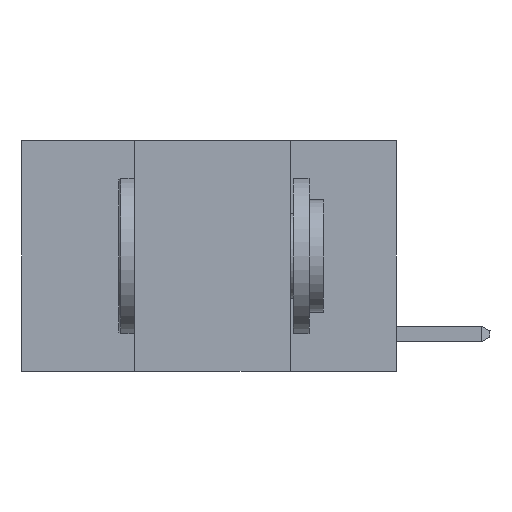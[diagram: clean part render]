
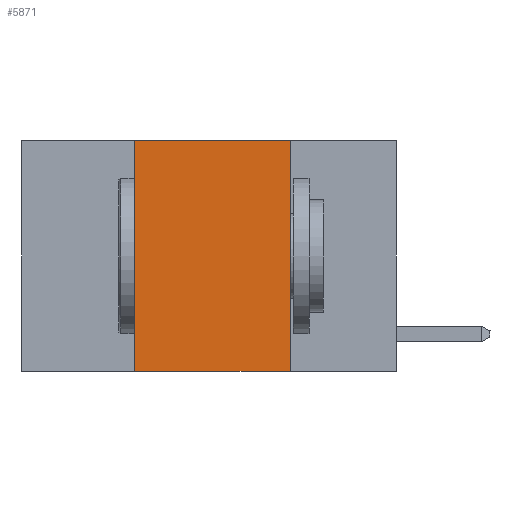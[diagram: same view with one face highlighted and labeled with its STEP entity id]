
A CAD part, left-side view. The second image highlights one B-rep face of the part: STEP entity #5871.
In plain terms, the highlighted planar face has unit normal (-1, 0, 0).
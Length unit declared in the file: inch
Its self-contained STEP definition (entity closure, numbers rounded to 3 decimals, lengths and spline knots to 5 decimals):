
#1015 = CARTESIAN_POINT ( 'NONE',  ( 0., 0.6, 0. ) ) ;
#1461 = EDGE_CURVE ( 'NONE', #13254, #6928, #4070, .T. ) ;
#3207 = ORIENTED_EDGE ( 'NONE', *, *, #6467, .F. ) ;
#3980 = VECTOR ( 'NONE', #6925, 39.37008 ) ;
#4070 = LINE ( 'NONE', #16595, #17649 ) ;
#4113 = VERTEX_POINT ( 'NONE', #13741 ) ;
#4834 = EDGE_CURVE ( 'NONE', #11380, #4113, #10329, .T. ) ;
#4855 = DIRECTION ( 'NONE',  ( 0., 0., -1. ) ) ;
#5230 = FACE_OUTER_BOUND ( 'NONE', #17068, .T. ) ;
#5660 = CARTESIAN_POINT ( 'NONE',  ( 0., 0.6, -0.37 ) ) ;
#5871 = ADVANCED_FACE ( 'NONE', ( #5230 ), #15273, .F. ) ;
#6467 = EDGE_CURVE ( 'NONE', #6928, #11380, #8586, .T. ) ;
#6522 = DIRECTION ( 'NONE',  ( 0., 0., 1. ) ) ;
#6925 = DIRECTION ( 'NONE',  ( 0., -1., 0. ) ) ;
#6928 = VERTEX_POINT ( 'NONE', #8847 ) ;
#7103 = CARTESIAN_POINT ( 'NONE',  ( 0., 0.6, 0. ) ) ;
#8586 = LINE ( 'NONE', #7103, #3980 ) ;
#8847 = CARTESIAN_POINT ( 'NONE',  ( 0., 0.42, 0. ) ) ;
#9042 = ORIENTED_EDGE ( 'NONE', *, *, #4834, .F. ) ;
#9173 = CARTESIAN_POINT ( 'NONE',  ( 0., 0.42, -0.37 ) ) ;
#10329 = LINE ( 'NONE', #13336, #13408 ) ;
#10881 = DIRECTION ( 'NONE',  ( 1., 0., 0. ) ) ;
#11380 = VERTEX_POINT ( 'NONE', #12838 ) ;
#12838 = CARTESIAN_POINT ( 'NONE',  ( 0., 0.17, 0. ) ) ;
#13044 = ORIENTED_EDGE ( 'NONE', *, *, #1461, .F. ) ;
#13254 = VERTEX_POINT ( 'NONE', #9173 ) ;
#13336 = CARTESIAN_POINT ( 'NONE',  ( 0., 0.17, 0. ) ) ;
#13408 = VECTOR ( 'NONE', #4855, 39.37008 ) ;
#13491 = AXIS2_PLACEMENT_3D ( 'NONE', #1015, #10881, #17850 ) ;
#13741 = CARTESIAN_POINT ( 'NONE',  ( 0., 0.17, -0.37 ) ) ;
#13793 = DIRECTION ( 'NONE',  ( 0., -1., 0. ) ) ;
#14468 = ORIENTED_EDGE ( 'NONE', *, *, #15325, .T. ) ;
#14841 = VECTOR ( 'NONE', #13793, 39.37008 ) ;
#15273 = PLANE ( 'NONE',  #13491 ) ;
#15325 = EDGE_CURVE ( 'NONE', #13254, #4113, #15446, .T. ) ;
#15446 = LINE ( 'NONE', #5660, #14841 ) ;
#16595 = CARTESIAN_POINT ( 'NONE',  ( 0., 0.42, 0. ) ) ;
#17068 = EDGE_LOOP ( 'NONE', ( #9042, #3207, #13044, #14468 ) ) ;
#17649 = VECTOR ( 'NONE', #6522, 39.37008 ) ;
#17850 = DIRECTION ( 'NONE',  ( 0., 0., -1. ) ) ;
